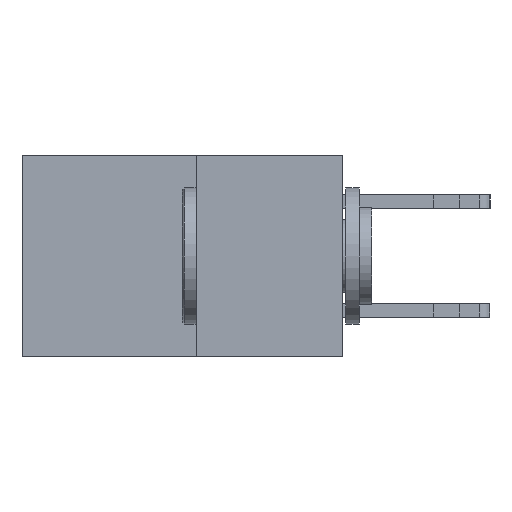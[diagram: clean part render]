
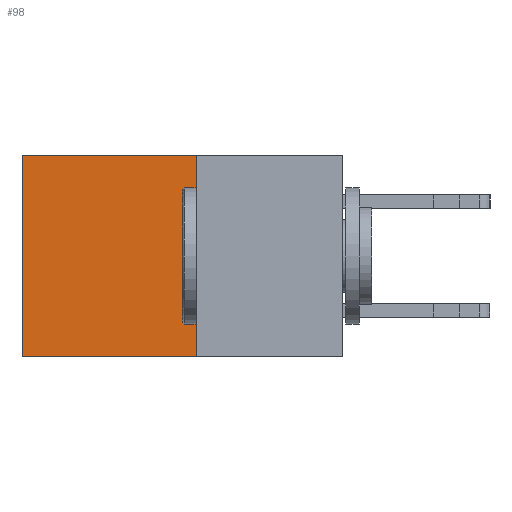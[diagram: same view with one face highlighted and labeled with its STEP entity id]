
A CAD part, left-side view. The second image highlights one B-rep face of the part: STEP entity #98.
In plain terms, the highlighted planar face has unit normal (-1, 0, 0).
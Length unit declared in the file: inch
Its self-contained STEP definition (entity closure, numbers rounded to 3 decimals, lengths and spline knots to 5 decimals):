
#98 = ADVANCED_FACE ( 'NONE', ( #27379 ), #21201, .F. ) ;
#1031 = VERTEX_POINT ( 'NONE', #9875 ) ;
#1288 = ORIENTED_EDGE ( 'NONE', *, *, #4158, .F. ) ;
#1662 = DIRECTION ( 'NONE',  ( 1., 0., 0. ) ) ;
#2698 = CARTESIAN_POINT ( 'NONE',  ( 0.277, 0.59, -0.37 ) ) ;
#2730 = EDGE_CURVE ( 'NONE', #19795, #13764, #31911, .T. ) ;
#3435 = EDGE_CURVE ( 'NONE', #1031, #19795, #4278, .T. ) ;
#4158 = EDGE_CURVE ( 'NONE', #1031, #17150, #7789, .T. ) ;
#4278 = LINE ( 'NONE', #24059, #10200 ) ;
#6307 = VECTOR ( 'NONE', #16014, 39.37008 ) ;
#6795 = CARTESIAN_POINT ( 'NONE',  ( 0.277, 0.59, -0.37 ) ) ;
#7789 = LINE ( 'NONE', #26925, #12163 ) ;
#9531 = LINE ( 'NONE', #15234, #10307 ) ;
#9732 = EDGE_LOOP ( 'NONE', ( #29919, #15831, #1288, #14406 ) ) ;
#9875 = CARTESIAN_POINT ( 'NONE',  ( 0.277, 0.27, 0. ) ) ;
#10200 = VECTOR ( 'NONE', #24085, 39.37008 ) ;
#10307 = VECTOR ( 'NONE', #28538, 39.37008 ) ;
#11900 = EDGE_CURVE ( 'NONE', #17150, #13764, #9531, .T. ) ;
#12163 = VECTOR ( 'NONE', #26639, 39.37008 ) ;
#13764 = VERTEX_POINT ( 'NONE', #6795 ) ;
#14406 = ORIENTED_EDGE ( 'NONE', *, *, #3435, .T. ) ;
#15234 = CARTESIAN_POINT ( 'NONE',  ( 0.277, 0.27, -0.37 ) ) ;
#15261 = CARTESIAN_POINT ( 'NONE',  ( 0.277, 0.27, -0.37 ) ) ;
#15689 = DIRECTION ( 'NONE',  ( 0., 0., -1. ) ) ;
#15831 = ORIENTED_EDGE ( 'NONE', *, *, #11900, .F. ) ;
#16014 = DIRECTION ( 'NONE',  ( 0., 0., -1. ) ) ;
#16381 = CARTESIAN_POINT ( 'NONE',  ( 0.277, 0.59, 0. ) ) ;
#17150 = VERTEX_POINT ( 'NONE', #19528 ) ;
#18334 = AXIS2_PLACEMENT_3D ( 'NONE', #15261, #1662, #15689 ) ;
#19528 = CARTESIAN_POINT ( 'NONE',  ( 0.277, 0.27, -0.37 ) ) ;
#19795 = VERTEX_POINT ( 'NONE', #16381 ) ;
#21201 = PLANE ( 'NONE',  #18334 ) ;
#24059 = CARTESIAN_POINT ( 'NONE',  ( 0.277, 0.27, 0. ) ) ;
#24085 = DIRECTION ( 'NONE',  ( 0., 1., 0. ) ) ;
#26639 = DIRECTION ( 'NONE',  ( 0., 0., -1. ) ) ;
#26925 = CARTESIAN_POINT ( 'NONE',  ( 0.277, 0.27, -0.37 ) ) ;
#27379 = FACE_OUTER_BOUND ( 'NONE', #9732, .T. ) ;
#28538 = DIRECTION ( 'NONE',  ( 0., 1., 0. ) ) ;
#29919 = ORIENTED_EDGE ( 'NONE', *, *, #2730, .T. ) ;
#31911 = LINE ( 'NONE', #2698, #6307 ) ;
